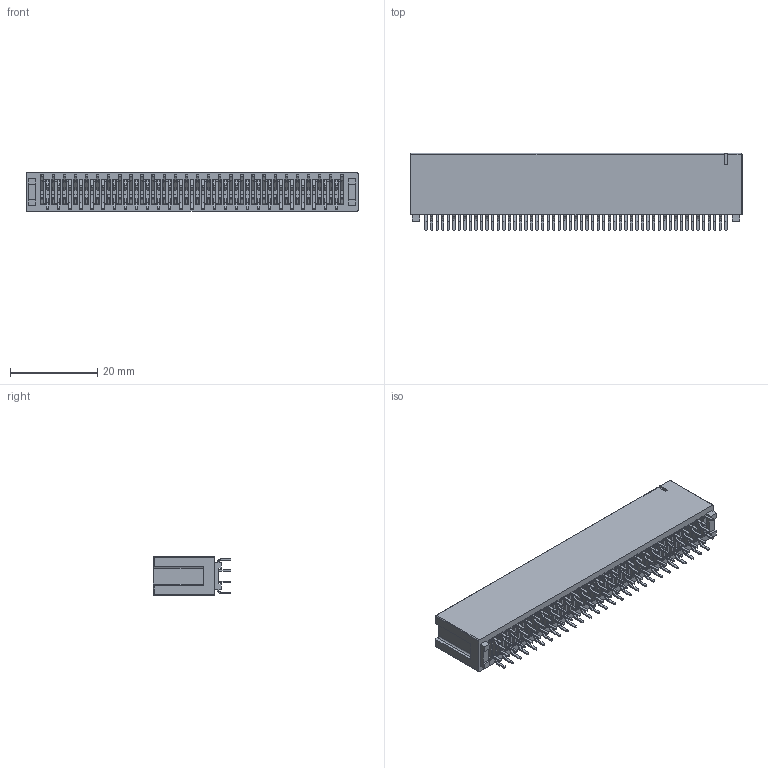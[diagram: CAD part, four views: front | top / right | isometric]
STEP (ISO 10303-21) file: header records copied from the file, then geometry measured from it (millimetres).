
FILE_DESCRIPTION (( 'STEP AP203' ), '1' );
FILE_NAME ('302-110-321-201.STEP', '2024-04-01T19:36:28', ( '' ), ( '' ), 'SwSTEP 2.0', 'SolidWorks 2023', '' );
FILE_SCHEMA (( 'CONFIG_CONTROL_DESIGN' ));
Length unit declared in the file: millimetre
Products named in the file (4): 302-110-321-201; Contact_302-290-X21 (2); Contact_302-290-X21 (1); HSG_Vertical HSG
Assembly tree (111 placements, depth 2):
  302-110-321-201
    HSG_Vertical HSG
    Contact_302-290-X21 (2)  x55
    Contact_302-290-X21 (1)  x55
Bounding box: 75.95 x 17.63 x 8.88 mm (x, y, z)
Volume: 5789.1 mm3; surface area: 16510.3 mm2
Topology: 111 solids, 111 shells, 5071 faces, 14908 edges, 9784 vertices
Faces by surface type: plane 3734, cylinder 1113, bspline 220, sphere 4
Entity records: 42686 total; most frequent: ORIENTED_EDGE 7344, CARTESIAN_POINT 7297, DIRECTION 5884, EDGE_CURVE 3672, VECTOR 3598, LINE 3598, VERTEX_POINT 2440, AXIS2_PLACEMENT_3D 1143
